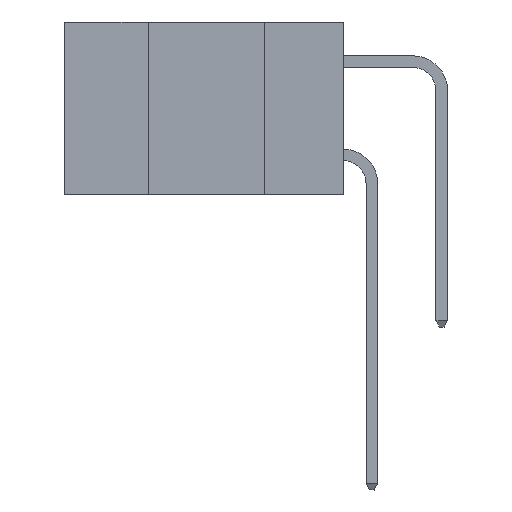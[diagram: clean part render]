
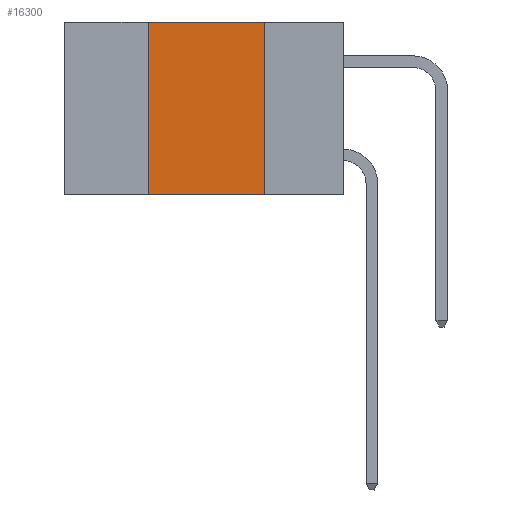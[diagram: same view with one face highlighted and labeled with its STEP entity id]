
A CAD part, left-side view. The second image highlights one B-rep face of the part: STEP entity #16300.
In plain terms, the highlighted planar face has unit normal (-1, 0, 0).
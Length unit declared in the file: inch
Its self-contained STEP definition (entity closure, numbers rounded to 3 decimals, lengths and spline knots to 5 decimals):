
#350 = LINE ( 'NONE', #24720, #24868 ) ;
#1923 = LINE ( 'NONE', #17934, #16932 ) ;
#2237 = ORIENTED_EDGE ( 'NONE', *, *, #11371, .F. ) ;
#2574 = VERTEX_POINT ( 'NONE', #15733 ) ;
#2582 = DIRECTION ( 'NONE',  ( 0., 0., -1. ) ) ;
#3130 = EDGE_CURVE ( 'NONE', #17296, #18355, #350, .T. ) ;
#3559 = VECTOR ( 'NONE', #14232, 39.37008 ) ;
#4557 = CARTESIAN_POINT ( 'NONE',  ( 0., 0.6, 0. ) ) ;
#4997 = ORIENTED_EDGE ( 'NONE', *, *, #16471, .F. ) ;
#5194 = AXIS2_PLACEMENT_3D ( 'NONE', #4557, #20562, #2582 ) ;
#5393 = CARTESIAN_POINT ( 'NONE',  ( 0., 0.42, -0.37 ) ) ;
#5492 = DIRECTION ( 'NONE',  ( 0., 0., -1. ) ) ;
#8321 = CARTESIAN_POINT ( 'NONE',  ( 0., 0.6, 0. ) ) ;
#11304 = VECTOR ( 'NONE', #5492, 39.37008 ) ;
#11371 = EDGE_CURVE ( 'NONE', #14181, #18355, #11403, .T. ) ;
#11403 = LINE ( 'NONE', #23726, #11304 ) ;
#11837 = ORIENTED_EDGE ( 'NONE', *, *, #3130, .T. ) ;
#13891 = ORIENTED_EDGE ( 'NONE', *, *, #25299, .F. ) ;
#14181 = VERTEX_POINT ( 'NONE', #22460 ) ;
#14232 = DIRECTION ( 'NONE',  ( 0., -1., 0. ) ) ;
#14354 = LINE ( 'NONE', #8321, #3559 ) ;
#15733 = CARTESIAN_POINT ( 'NONE',  ( 0., 0.42, 0. ) ) ;
#16300 = ADVANCED_FACE ( 'NONE', ( #22533 ), #18600, .F. ) ;
#16350 = DIRECTION ( 'NONE',  ( 0., -1., 0. ) ) ;
#16471 = EDGE_CURVE ( 'NONE', #17296, #2574, #1923, .T. ) ;
#16932 = VECTOR ( 'NONE', #18057, 39.37008 ) ;
#17296 = VERTEX_POINT ( 'NONE', #5393 ) ;
#17934 = CARTESIAN_POINT ( 'NONE',  ( 0., 0.42, -0.37 ) ) ;
#18057 = DIRECTION ( 'NONE',  ( 0., 0., 1. ) ) ;
#18355 = VERTEX_POINT ( 'NONE', #19266 ) ;
#18600 = PLANE ( 'NONE',  #5194 ) ;
#18622 = EDGE_LOOP ( 'NONE', ( #2237, #13891, #4997, #11837 ) ) ;
#19266 = CARTESIAN_POINT ( 'NONE',  ( 0., 0.17, -0.37 ) ) ;
#20562 = DIRECTION ( 'NONE',  ( 1., 0., 0. ) ) ;
#22460 = CARTESIAN_POINT ( 'NONE',  ( 0., 0.17, 0. ) ) ;
#22533 = FACE_OUTER_BOUND ( 'NONE', #18622, .T. ) ;
#23726 = CARTESIAN_POINT ( 'NONE',  ( 0., 0.17, -0.37 ) ) ;
#24720 = CARTESIAN_POINT ( 'NONE',  ( 0., 0.6, -0.37 ) ) ;
#24868 = VECTOR ( 'NONE', #16350, 39.37008 ) ;
#25299 = EDGE_CURVE ( 'NONE', #2574, #14181, #14354, .T. ) ;
